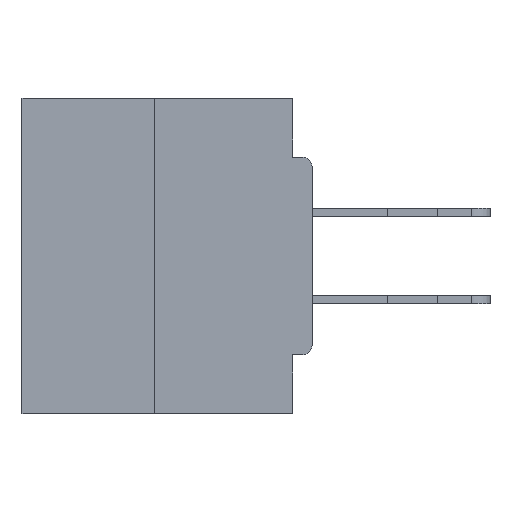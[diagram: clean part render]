
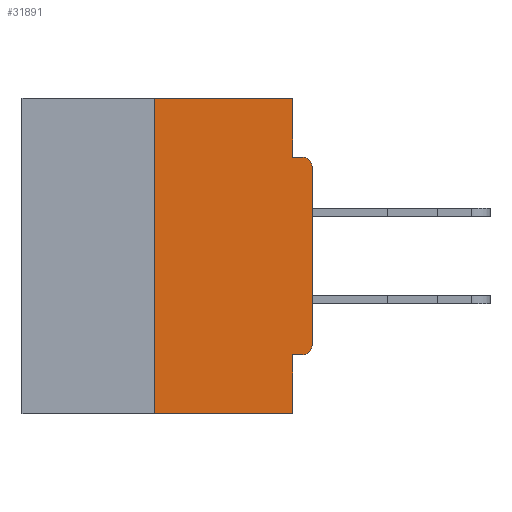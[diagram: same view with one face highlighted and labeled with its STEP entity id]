
A CAD part, left-side view. The second image highlights one B-rep face of the part: STEP entity #31891.
In plain terms, the highlighted planar face has unit normal (-1, 0, 0).
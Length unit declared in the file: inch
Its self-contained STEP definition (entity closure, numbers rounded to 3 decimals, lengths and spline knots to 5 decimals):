
#656 = VECTOR ( 'NONE', #26241, 39.37008 ) ;
#1423 = LINE ( 'NONE', #33168, #22044 ) ;
#1554 = LINE ( 'NONE', #7185, #12436 ) ;
#2111 = DIRECTION ( 'NONE',  ( 0., -1., 0. ) ) ;
#2810 = AXIS2_PLACEMENT_3D ( 'NONE', #19893, #9941, #4640 ) ;
#3236 = LINE ( 'NONE', #26474, #14532 ) ;
#3242 = LINE ( 'NONE', #18073, #5251 ) ;
#3293 = CARTESIAN_POINT ( 'NONE',  ( 0., 0.031, -0.5 ) ) ;
#3316 = VERTEX_POINT ( 'NONE', #21614 ) ;
#4640 = DIRECTION ( 'NONE',  ( 0., 0., -1. ) ) ;
#5251 = VECTOR ( 'NONE', #10039, 39.37008 ) ;
#5683 = DIRECTION ( 'NONE',  ( 0., 0., 1. ) ) ;
#5892 = EDGE_CURVE ( 'NONE', #15654, #11219, #3242, .T. ) ;
#6173 = CARTESIAN_POINT ( 'NONE',  ( 0., 0.25, 0. ) ) ;
#7185 = CARTESIAN_POINT ( 'NONE',  ( 0., 0., -0.0935 ) ) ;
#8465 = EDGE_CURVE ( 'NONE', #29503, #11219, #14389, .T. ) ;
#8467 = DIRECTION ( 'NONE',  ( 0., 0., -1. ) ) ;
#8889 = EDGE_CURVE ( 'NONE', #29503, #32654, #15675, .T. ) ;
#8996 = CARTESIAN_POINT ( 'NONE',  ( 0., 0., -0.3915 ) ) ;
#9228 = CIRCLE ( 'NONE', #19168, 0.015 ) ;
#9853 = VERTEX_POINT ( 'NONE', #30826 ) ;
#9941 = DIRECTION ( 'NONE',  ( 1., 0., 0. ) ) ;
#10039 = DIRECTION ( 'NONE',  ( 0., 0., -1. ) ) ;
#11219 = VERTEX_POINT ( 'NONE', #3293 ) ;
#11264 = CARTESIAN_POINT ( 'NONE',  ( 0., 0.031, -0.0935 ) ) ;
#12109 = EDGE_CURVE ( 'NONE', #3316, #15124, #24224, .T. ) ;
#12436 = VECTOR ( 'NONE', #2111, 39.37008 ) ;
#13278 = CIRCLE ( 'NONE', #20496, 0.015 ) ;
#14389 = LINE ( 'NONE', #32747, #32562 ) ;
#14532 = VECTOR ( 'NONE', #5683, 39.37008 ) ;
#14621 = ORIENTED_EDGE ( 'NONE', *, *, #8465, .T. ) ;
#15124 = VERTEX_POINT ( 'NONE', #11264 ) ;
#15641 = EDGE_LOOP ( 'NONE', ( #27074, #23747, #14621, #17597, #25172, #32429, #24213, #25082, #30671, #29741 ) ) ;
#15654 = VERTEX_POINT ( 'NONE', #32198 ) ;
#15675 = LINE ( 'NONE', #26127, #656 ) ;
#16738 = EDGE_CURVE ( 'NONE', #23444, #15654, #1423, .T. ) ;
#17597 = ORIENTED_EDGE ( 'NONE', *, *, #5892, .F. ) ;
#18073 = CARTESIAN_POINT ( 'NONE',  ( 0., 0.031, -0.5 ) ) ;
#18121 = DIRECTION ( 'NONE',  ( 0., -1., 0. ) ) ;
#19168 = AXIS2_PLACEMENT_3D ( 'NONE', #28536, #26398, #21331 ) ;
#19483 = VERTEX_POINT ( 'NONE', #32684 ) ;
#19893 = CARTESIAN_POINT ( 'NONE',  ( 0., 0.46, 0. ) ) ;
#20480 = CARTESIAN_POINT ( 'NONE',  ( 0., 0.25, -0.5 ) ) ;
#20496 = AXIS2_PLACEMENT_3D ( 'NONE', #21441, #31918, #29439 ) ;
#21331 = DIRECTION ( 'NONE',  ( 0., 0., -1. ) ) ;
#21441 = CARTESIAN_POINT ( 'NONE',  ( 0., 0.015, -0.3915 ) ) ;
#21614 = CARTESIAN_POINT ( 'NONE',  ( 0., 0.031, 0. ) ) ;
#22044 = VECTOR ( 'NONE', #22808, 39.37008 ) ;
#22808 = DIRECTION ( 'NONE',  ( 0., 1., 0. ) ) ;
#23324 = CARTESIAN_POINT ( 'NONE',  ( 0., 0.46, 0. ) ) ;
#23444 = VERTEX_POINT ( 'NONE', #26846 ) ;
#23747 = ORIENTED_EDGE ( 'NONE', *, *, #8889, .F. ) ;
#23973 = CARTESIAN_POINT ( 'NONE',  ( 0., 0.031, 0. ) ) ;
#24213 = ORIENTED_EDGE ( 'NONE', *, *, #25474, .T. ) ;
#24224 = LINE ( 'NONE', #23973, #29059 ) ;
#25023 = VERTEX_POINT ( 'NONE', #8996 ) ;
#25080 = EDGE_CURVE ( 'NONE', #32654, #3316, #26697, .T. ) ;
#25082 = ORIENTED_EDGE ( 'NONE', *, *, #26613, .T. ) ;
#25172 = ORIENTED_EDGE ( 'NONE', *, *, #16738, .F. ) ;
#25474 = EDGE_CURVE ( 'NONE', #25023, #9853, #3236, .T. ) ;
#26127 = CARTESIAN_POINT ( 'NONE',  ( 0., 0.25, 0. ) ) ;
#26241 = DIRECTION ( 'NONE',  ( 0., 0., 1. ) ) ;
#26327 = EDGE_CURVE ( 'NONE', #15124, #19483, #1554, .T. ) ;
#26398 = DIRECTION ( 'NONE',  ( -1., 0., 0. ) ) ;
#26474 = CARTESIAN_POINT ( 'NONE',  ( 0., 0., 0. ) ) ;
#26613 = EDGE_CURVE ( 'NONE', #9853, #19483, #9228, .T. ) ;
#26697 = LINE ( 'NONE', #23324, #30744 ) ;
#26846 = CARTESIAN_POINT ( 'NONE',  ( 0., 0.015, -0.4065 ) ) ;
#27074 = ORIENTED_EDGE ( 'NONE', *, *, #25080, .F. ) ;
#27356 = DIRECTION ( 'NONE',  ( 0., -1., 0. ) ) ;
#28012 = FACE_OUTER_BOUND ( 'NONE', #15641, .T. ) ;
#28132 = EDGE_CURVE ( 'NONE', #23444, #25023, #13278, .T. ) ;
#28536 = CARTESIAN_POINT ( 'NONE',  ( 0., 0.015, -0.1085 ) ) ;
#29059 = VECTOR ( 'NONE', #8467, 39.37008 ) ;
#29439 = DIRECTION ( 'NONE',  ( 0., 0., -1. ) ) ;
#29503 = VERTEX_POINT ( 'NONE', #20480 ) ;
#29741 = ORIENTED_EDGE ( 'NONE', *, *, #12109, .F. ) ;
#30671 = ORIENTED_EDGE ( 'NONE', *, *, #26327, .F. ) ;
#30744 = VECTOR ( 'NONE', #18121, 39.37008 ) ;
#30826 = CARTESIAN_POINT ( 'NONE',  ( 0., 0., -0.1085 ) ) ;
#31891 = ADVANCED_FACE ( 'NONE', ( #28012 ), #32864, .F. ) ;
#31918 = DIRECTION ( 'NONE',  ( -1., 0., 0. ) ) ;
#32198 = CARTESIAN_POINT ( 'NONE',  ( 0., 0.031, -0.4065 ) ) ;
#32429 = ORIENTED_EDGE ( 'NONE', *, *, #28132, .T. ) ;
#32562 = VECTOR ( 'NONE', #27356, 39.37008 ) ;
#32654 = VERTEX_POINT ( 'NONE', #6173 ) ;
#32684 = CARTESIAN_POINT ( 'NONE',  ( 0., 0.015, -0.0935 ) ) ;
#32747 = CARTESIAN_POINT ( 'NONE',  ( 0., 0.46, -0.5 ) ) ;
#32864 = PLANE ( 'NONE',  #2810 ) ;
#33168 = CARTESIAN_POINT ( 'NONE',  ( 0., 0., -0.4065 ) ) ;
